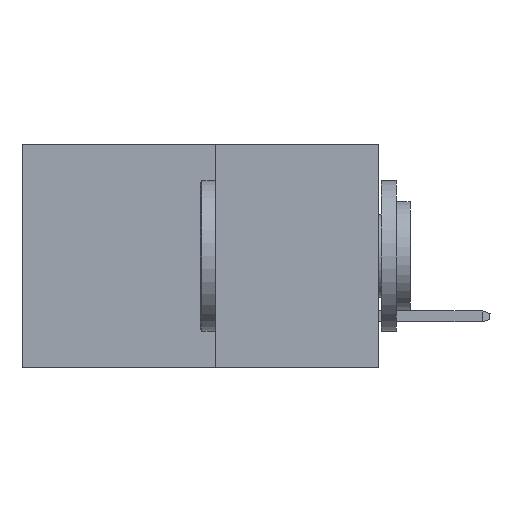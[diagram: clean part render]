
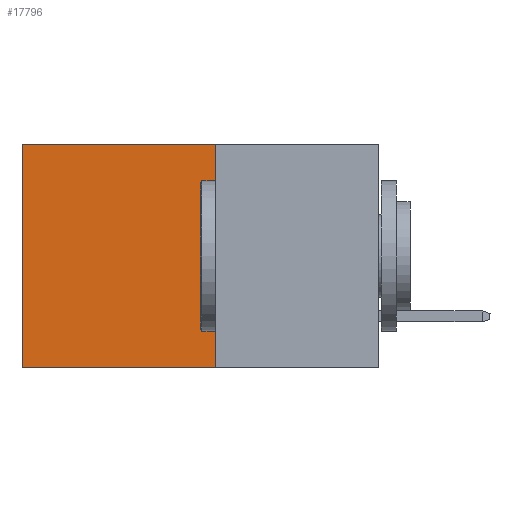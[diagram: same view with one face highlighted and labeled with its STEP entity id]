
A CAD part, left-side view. The second image highlights one B-rep face of the part: STEP entity #17796.
In plain terms, the highlighted planar face has unit normal (-1, 0, 0).
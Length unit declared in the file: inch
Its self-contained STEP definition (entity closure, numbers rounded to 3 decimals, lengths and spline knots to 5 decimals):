
#230 = VERTEX_POINT ( 'NONE', #12540 ) ;
#2116 = DIRECTION ( 'NONE',  ( 0., 1., 0. ) ) ;
#2117 = VECTOR ( 'NONE', #5370, 39.37008 ) ;
#3677 = ORIENTED_EDGE ( 'NONE', *, *, #5235, .T. ) ;
#4168 = EDGE_LOOP ( 'NONE', ( #3677, #17801, #22139, #10189 ) ) ;
#5235 = EDGE_CURVE ( 'NONE', #14697, #230, #25185, .T. ) ;
#5370 = DIRECTION ( 'NONE',  ( 0., 1., 0. ) ) ;
#7094 = LINE ( 'NONE', #18469, #11869 ) ;
#8406 = DIRECTION ( 'NONE',  ( 1., 0., 0. ) ) ;
#10189 = ORIENTED_EDGE ( 'NONE', *, *, #14208, .T. ) ;
#10200 = AXIS2_PLACEMENT_3D ( 'NONE', #12423, #8406, #22630 ) ;
#11195 = CARTESIAN_POINT ( 'NONE',  ( 0.277, 0.27, 0. ) ) ;
#11304 = CARTESIAN_POINT ( 'NONE',  ( 0.277, 0.27, -0.37 ) ) ;
#11869 = VECTOR ( 'NONE', #2116, 39.37008 ) ;
#11922 = CARTESIAN_POINT ( 'NONE',  ( 0.277, 0.59, 0. ) ) ;
#12423 = CARTESIAN_POINT ( 'NONE',  ( 0.277, 0.27, -0.37 ) ) ;
#12540 = CARTESIAN_POINT ( 'NONE',  ( 0.277, 0.59, -0.37 ) ) ;
#13887 = DIRECTION ( 'NONE',  ( 0., 0., -1. ) ) ;
#14208 = EDGE_CURVE ( 'NONE', #20266, #14697, #7094, .T. ) ;
#14697 = VERTEX_POINT ( 'NONE', #11922 ) ;
#15333 = EDGE_CURVE ( 'NONE', #20266, #25401, #26044, .T. ) ;
#15571 = CARTESIAN_POINT ( 'NONE',  ( 0.277, 0.27, -0.37 ) ) ;
#15776 = VECTOR ( 'NONE', #22640, 39.37008 ) ;
#15857 = CARTESIAN_POINT ( 'NONE',  ( 0.277, 0.27, -0.37 ) ) ;
#17796 = ADVANCED_FACE ( 'NONE', ( #18427 ), #18592, .F. ) ;
#17801 = ORIENTED_EDGE ( 'NONE', *, *, #21031, .F. ) ;
#18426 = LINE ( 'NONE', #15571, #2117 ) ;
#18427 = FACE_OUTER_BOUND ( 'NONE', #4168, .T. ) ;
#18469 = CARTESIAN_POINT ( 'NONE',  ( 0.277, 0.27, 0. ) ) ;
#18592 = PLANE ( 'NONE',  #10200 ) ;
#20266 = VERTEX_POINT ( 'NONE', #11195 ) ;
#20790 = VECTOR ( 'NONE', #13887, 39.37008 ) ;
#21031 = EDGE_CURVE ( 'NONE', #25401, #230, #18426, .T. ) ;
#22139 = ORIENTED_EDGE ( 'NONE', *, *, #15333, .F. ) ;
#22630 = DIRECTION ( 'NONE',  ( 0., 0., -1. ) ) ;
#22640 = DIRECTION ( 'NONE',  ( 0., 0., -1. ) ) ;
#23272 = CARTESIAN_POINT ( 'NONE',  ( 0.277, 0.59, -0.37 ) ) ;
#25185 = LINE ( 'NONE', #23272, #15776 ) ;
#25401 = VERTEX_POINT ( 'NONE', #11304 ) ;
#26044 = LINE ( 'NONE', #15857, #20790 ) ;
